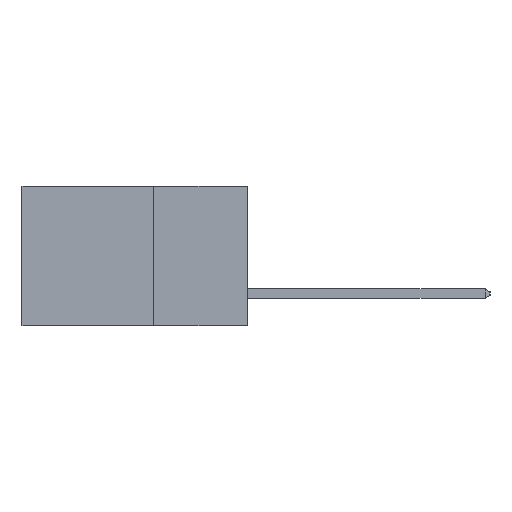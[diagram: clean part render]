
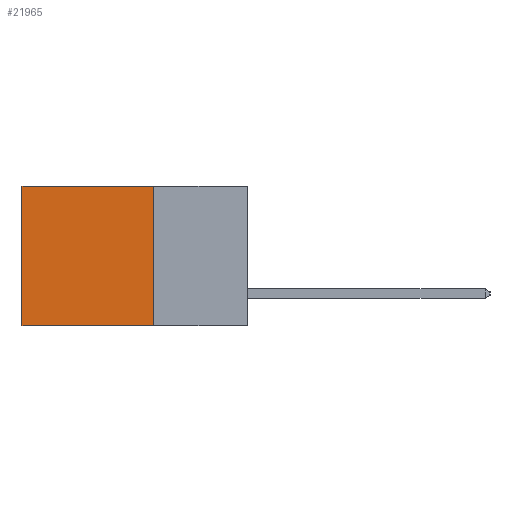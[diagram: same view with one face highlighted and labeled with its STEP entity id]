
A CAD part, left-side view. The second image highlights one B-rep face of the part: STEP entity #21965.
In plain terms, the highlighted planar face has unit normal (-1, 0, 0).
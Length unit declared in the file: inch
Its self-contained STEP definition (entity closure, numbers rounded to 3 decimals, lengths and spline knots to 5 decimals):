
#14 = CARTESIAN_POINT ( 'NONE',  ( 0.2615, 0.25, -0.37 ) ) ;
#1047 = VERTEX_POINT ( 'NONE', #15474 ) ;
#2364 = AXIS2_PLACEMENT_3D ( 'NONE', #9266, #21078, #11022 ) ;
#4075 = CARTESIAN_POINT ( 'NONE',  ( 0.2615, 0.6, -0.37 ) ) ;
#4700 = LINE ( 'NONE', #9866, #8264 ) ;
#6797 = DIRECTION ( 'NONE',  ( 0., 0., -1. ) ) ;
#6879 = ORIENTED_EDGE ( 'NONE', *, *, #16603, .T. ) ;
#6893 = ORIENTED_EDGE ( 'NONE', *, *, #9045, .F. ) ;
#7053 = CARTESIAN_POINT ( 'NONE',  ( 0.2615, 0.6, -0.37 ) ) ;
#7344 = VECTOR ( 'NONE', #17707, 39.37008 ) ;
#8264 = VECTOR ( 'NONE', #21615, 39.37008 ) ;
#9045 = EDGE_CURVE ( 'NONE', #1047, #15787, #15338, .T. ) ;
#9223 = VERTEX_POINT ( 'NONE', #15199 ) ;
#9240 = ORIENTED_EDGE ( 'NONE', *, *, #13645, .T. ) ;
#9266 = CARTESIAN_POINT ( 'NONE',  ( 0.2615, 0.25, -0.37 ) ) ;
#9506 = CARTESIAN_POINT ( 'NONE',  ( 0.2615, 0.25, -0.37 ) ) ;
#9853 = LINE ( 'NONE', #14, #17796 ) ;
#9866 = CARTESIAN_POINT ( 'NONE',  ( 0.2615, 0.25, 0. ) ) ;
#10665 = FACE_OUTER_BOUND ( 'NONE', #15134, .T. ) ;
#11022 = DIRECTION ( 'NONE',  ( 0., 0., -1. ) ) ;
#11439 = VECTOR ( 'NONE', #6797, 39.37008 ) ;
#13645 = EDGE_CURVE ( 'NONE', #16557, #15787, #20409, .T. ) ;
#15134 = EDGE_LOOP ( 'NONE', ( #9240, #6893, #20309, #6879 ) ) ;
#15199 = CARTESIAN_POINT ( 'NONE',  ( 0.2615, 0.25, 0. ) ) ;
#15338 = LINE ( 'NONE', #9506, #7344 ) ;
#15474 = CARTESIAN_POINT ( 'NONE',  ( 0.2615, 0.25, -0.37 ) ) ;
#15787 = VERTEX_POINT ( 'NONE', #4075 ) ;
#16036 = PLANE ( 'NONE',  #2364 ) ;
#16557 = VERTEX_POINT ( 'NONE', #21548 ) ;
#16603 = EDGE_CURVE ( 'NONE', #9223, #16557, #4700, .T. ) ;
#17403 = EDGE_CURVE ( 'NONE', #9223, #1047, #9853, .T. ) ;
#17707 = DIRECTION ( 'NONE',  ( 0., 1., 0. ) ) ;
#17796 = VECTOR ( 'NONE', #18916, 39.37008 ) ;
#18916 = DIRECTION ( 'NONE',  ( 0., 0., -1. ) ) ;
#20309 = ORIENTED_EDGE ( 'NONE', *, *, #17403, .F. ) ;
#20409 = LINE ( 'NONE', #7053, #11439 ) ;
#21078 = DIRECTION ( 'NONE',  ( 1., 0., 0. ) ) ;
#21548 = CARTESIAN_POINT ( 'NONE',  ( 0.2615, 0.6, 0. ) ) ;
#21615 = DIRECTION ( 'NONE',  ( 0., 1., 0. ) ) ;
#21965 = ADVANCED_FACE ( 'NONE', ( #10665 ), #16036, .F. ) ;
